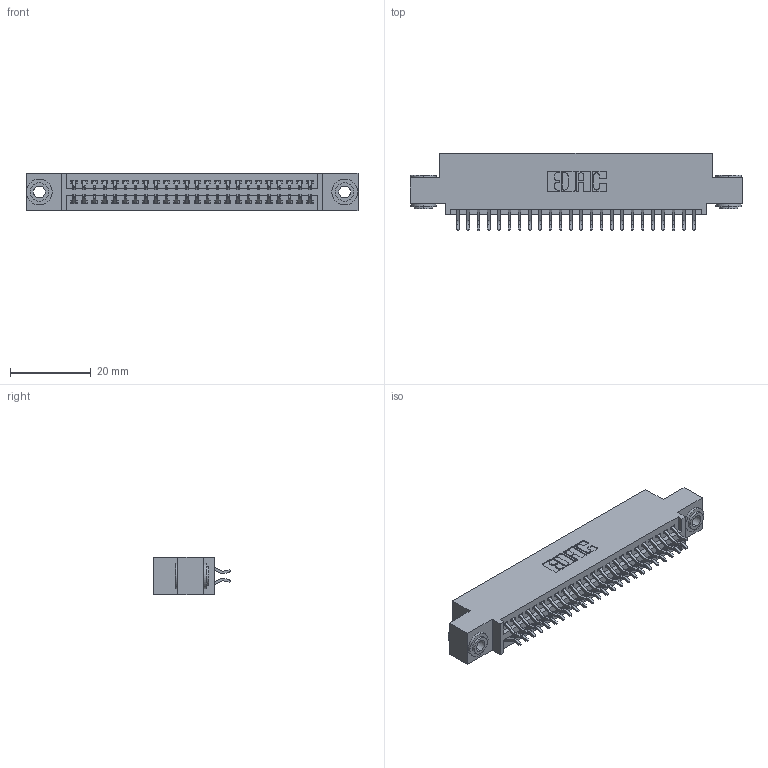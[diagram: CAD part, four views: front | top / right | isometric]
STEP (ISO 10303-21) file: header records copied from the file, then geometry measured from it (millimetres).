
FILE_DESCRIPTION (( 'STEP AP203' ), '1' );
FILE_NAME ('395-048-556-503.STEP', '2019-10-19T06:14:51', ( '' ), ( '' ), 'SwSTEP 2.0', 'SolidWorks 2016', '' );
FILE_SCHEMA (( 'CONFIG_CONTROL_DESIGN' ));
Length unit declared in the file: inch
Products named in the file (4): 345 Part_0.110 Offset - 0.156 Dia-TH; 345-292-001_556 Tail; 345-250-002_345-250-002-102; 395-048-556-503
Assembly tree (51 placements, depth 2):
  395-048-556-503
    345 Part_0.110 Offset - 0.156 Dia-TH
    345-292-001_556 Tail  x48
    345-250-002_345-250-002-102  x2
Bounding box: 82.17 x 19.24 x 9.4 mm (x, y, z)
Volume: 7759 mm3; surface area: 11376.2 mm2
Topology: 51 solids, 51 shells, 2856 faces, 8445 edges, 5562 vertices
Faces by surface type: plane 1870, cylinder 978, cone 8
Entity records: 22256 total; most frequent: CARTESIAN_POINT 3739, ORIENTED_EDGE 3654, DIRECTION 3337, EDGE_CURVE 1827, LINE 1567, VECTOR 1567, VERTEX_POINT 1214, AXIS2_PLACEMENT_3D 885
